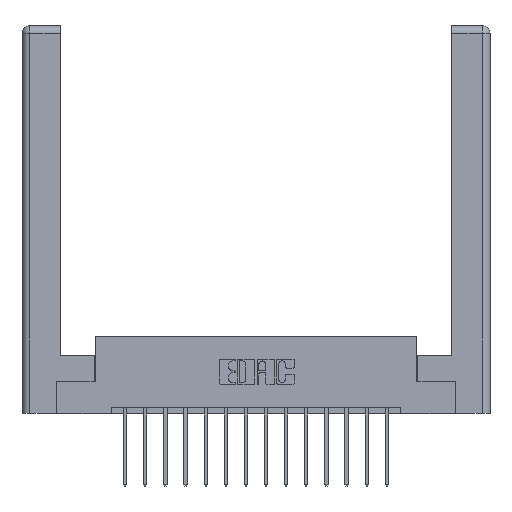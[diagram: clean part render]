
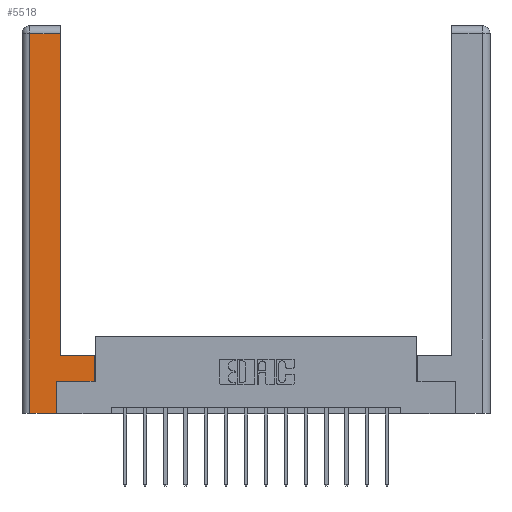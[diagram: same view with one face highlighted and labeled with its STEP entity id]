
A CAD part, top view. The second image highlights one B-rep face of the part: STEP entity #5518.
In plain terms, the highlighted planar face has unit normal (0, 0, 1).
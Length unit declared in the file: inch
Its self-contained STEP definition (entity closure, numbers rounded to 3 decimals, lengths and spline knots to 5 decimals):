
#110 = CARTESIAN_POINT ( 'NONE',  ( 0.565, 0.45, 0. ) ) ;
#578 = DIRECTION ( 'NONE',  ( -1., 0., 0. ) ) ;
#951 = CARTESIAN_POINT ( 'NONE',  ( 0.295, 0.45, 0. ) ) ;
#1284 = VERTEX_POINT ( 'NONE', #2321 ) ;
#1342 = ORIENTED_EDGE ( 'NONE', *, *, #2548, .T. ) ;
#1519 = DIRECTION ( 'NONE',  ( -1., 0., 0. ) ) ;
#1654 = LINE ( 'NONE', #15776, #15282 ) ;
#1717 = VERTEX_POINT ( 'NONE', #3869 ) ;
#2226 = LINE ( 'NONE', #10170, #12558 ) ;
#2320 = DIRECTION ( 'NONE',  ( 0., 1., 0. ) ) ;
#2321 = CARTESIAN_POINT ( 'NONE',  ( 0.265, 0., 0. ) ) ;
#2548 = EDGE_CURVE ( 'NONE', #9452, #1717, #9788, .T. ) ;
#2658 = VERTEX_POINT ( 'NONE', #951 ) ;
#2693 = VERTEX_POINT ( 'NONE', #3890 ) ;
#3143 = VERTEX_POINT ( 'NONE', #8467 ) ;
#3188 = EDGE_CURVE ( 'NONE', #1284, #7486, #9173, .T. ) ;
#3317 = ORIENTED_EDGE ( 'NONE', *, *, #14208, .T. ) ;
#3361 = LINE ( 'NONE', #6915, #13485 ) ;
#3869 = CARTESIAN_POINT ( 'NONE',  ( 0.565, 0.45, 0. ) ) ;
#3890 = CARTESIAN_POINT ( 'NONE',  ( 0.295, 2.94, 0. ) ) ;
#3943 = DIRECTION ( 'NONE',  ( 1., 0., 0. ) ) ;
#3964 = EDGE_CURVE ( 'NONE', #8446, #1284, #12005, .T. ) ;
#4023 = CARTESIAN_POINT ( 'NONE',  ( 0., 0., 0. ) ) ;
#4858 = EDGE_CURVE ( 'NONE', #2693, #3143, #15235, .T. ) ;
#5335 = DIRECTION ( 'NONE',  ( 1., 0., 0. ) ) ;
#5347 = DIRECTION ( 'NONE',  ( 0., 0., -1. ) ) ;
#5518 = ADVANCED_FACE ( 'NONE', ( #11944 ), #15078, .F. ) ;
#6043 = VECTOR ( 'NONE', #14166, 39.37008 ) ;
#6074 = ORIENTED_EDGE ( 'NONE', *, *, #10739, .T. ) ;
#6285 = VECTOR ( 'NONE', #15855, 39.37008 ) ;
#6915 = CARTESIAN_POINT ( 'NONE',  ( 0.295, 0.45, 0. ) ) ;
#7283 = ORIENTED_EDGE ( 'NONE', *, *, #11946, .T. ) ;
#7318 = CARTESIAN_POINT ( 'NONE',  ( 0.0615, 0., 0. ) ) ;
#7486 = VERTEX_POINT ( 'NONE', #16349 ) ;
#8073 = CARTESIAN_POINT ( 'NONE',  ( 0.265, 0., 0. ) ) ;
#8446 = VERTEX_POINT ( 'NONE', #7318 ) ;
#8467 = CARTESIAN_POINT ( 'NONE',  ( 0.0615, 2.94, 0. ) ) ;
#9173 = LINE ( 'NONE', #14052, #6043 ) ;
#9178 = CARTESIAN_POINT ( 'NONE',  ( 0.295, 3., 0. ) ) ;
#9452 = VERTEX_POINT ( 'NONE', #11548 ) ;
#9555 = DIRECTION ( 'NONE',  ( -1., 0., 0. ) ) ;
#9788 = LINE ( 'NONE', #110, #6285 ) ;
#10170 = CARTESIAN_POINT ( 'NONE',  ( 0.0615, 0., 0. ) ) ;
#10640 = LINE ( 'NONE', #9178, #15782 ) ;
#10647 = ORIENTED_EDGE ( 'NONE', *, *, #4858, .T. ) ;
#10739 = EDGE_CURVE ( 'NONE', #7486, #9452, #1654, .T. ) ;
#11078 = AXIS2_PLACEMENT_3D ( 'NONE', #4023, #5347, #1519 ) ;
#11548 = CARTESIAN_POINT ( 'NONE',  ( 0.565, 0.245, 0. ) ) ;
#11830 = ORIENTED_EDGE ( 'NONE', *, *, #13321, .T. ) ;
#11944 = FACE_OUTER_BOUND ( 'NONE', #16266, .T. ) ;
#11946 = EDGE_CURVE ( 'NONE', #3143, #8446, #2226, .T. ) ;
#12005 = LINE ( 'NONE', #8073, #14865 ) ;
#12236 = ORIENTED_EDGE ( 'NONE', *, *, #3188, .T. ) ;
#12558 = VECTOR ( 'NONE', #12696, 39.37008 ) ;
#12696 = DIRECTION ( 'NONE',  ( 0., -1., 0. ) ) ;
#13276 = ORIENTED_EDGE ( 'NONE', *, *, #3964, .T. ) ;
#13321 = EDGE_CURVE ( 'NONE', #2658, #2693, #10640, .T. ) ;
#13448 = CARTESIAN_POINT ( 'NONE',  ( 0.0615, 2.94, 0. ) ) ;
#13485 = VECTOR ( 'NONE', #9555, 39.37008 ) ;
#14052 = CARTESIAN_POINT ( 'NONE',  ( 0.265, 0.245, 0. ) ) ;
#14166 = DIRECTION ( 'NONE',  ( 0., 1., 0. ) ) ;
#14208 = EDGE_CURVE ( 'NONE', #1717, #2658, #3361, .T. ) ;
#14865 = VECTOR ( 'NONE', #3943, 39.37008 ) ;
#15078 = PLANE ( 'NONE',  #11078 ) ;
#15235 = LINE ( 'NONE', #13448, #15670 ) ;
#15282 = VECTOR ( 'NONE', #5335, 39.37008 ) ;
#15670 = VECTOR ( 'NONE', #578, 39.37008 ) ;
#15776 = CARTESIAN_POINT ( 'NONE',  ( 0.565, 0.245, 0. ) ) ;
#15782 = VECTOR ( 'NONE', #2320, 39.37008 ) ;
#15855 = DIRECTION ( 'NONE',  ( 0., 1., 0. ) ) ;
#16266 = EDGE_LOOP ( 'NONE', ( #11830, #10647, #7283, #13276, #12236, #6074, #1342, #3317 ) ) ;
#16349 = CARTESIAN_POINT ( 'NONE',  ( 0.265, 0.245, 0. ) ) ;
